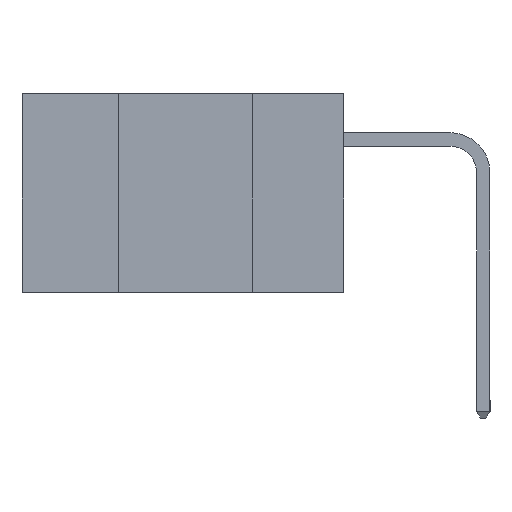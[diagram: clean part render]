
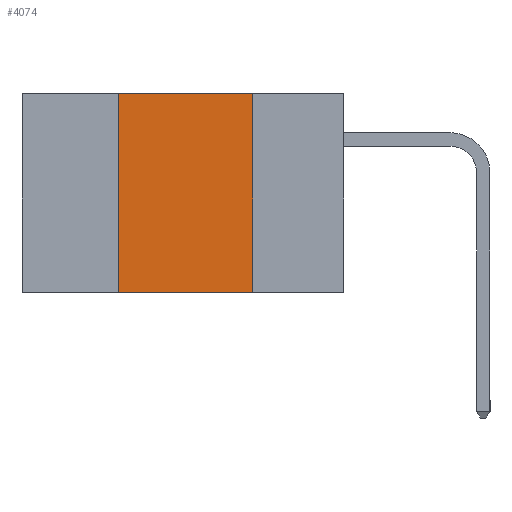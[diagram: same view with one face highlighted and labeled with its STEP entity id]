
A CAD part, left-side view. The second image highlights one B-rep face of the part: STEP entity #4074.
In plain terms, the highlighted planar face has unit normal (-1, 0, 0).
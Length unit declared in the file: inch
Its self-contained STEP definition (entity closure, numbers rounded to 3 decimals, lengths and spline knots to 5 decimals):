
#386 = VECTOR ( 'NONE', #10915, 39.37008 ) ;
#509 = VERTEX_POINT ( 'NONE', #4034 ) ;
#665 = CARTESIAN_POINT ( 'NONE',  ( 0., 0.6, 0. ) ) ;
#705 = ORIENTED_EDGE ( 'NONE', *, *, #10083, .F. ) ;
#811 = VECTOR ( 'NONE', #11705, 39.37008 ) ;
#926 = ORIENTED_EDGE ( 'NONE', *, *, #9241, .F. ) ;
#1350 = LINE ( 'NONE', #15082, #14401 ) ;
#3184 = VERTEX_POINT ( 'NONE', #14435 ) ;
#3360 = EDGE_LOOP ( 'NONE', ( #15332, #705, #926, #4141 ) ) ;
#3818 = LINE ( 'NONE', #4060, #811 ) ;
#4034 = CARTESIAN_POINT ( 'NONE',  ( 0., 0.42, 0. ) ) ;
#4060 = CARTESIAN_POINT ( 'NONE',  ( 0., 0.42, -0.37 ) ) ;
#4074 = ADVANCED_FACE ( 'NONE', ( #5512 ), #8255, .F. ) ;
#4141 = ORIENTED_EDGE ( 'NONE', *, *, #8368, .T. ) ;
#5512 = FACE_OUTER_BOUND ( 'NONE', #3360, .T. ) ;
#5934 = LINE ( 'NONE', #10351, #9000 ) ;
#8171 = DIRECTION ( 'NONE',  ( 0., 0., -1. ) ) ;
#8212 = CARTESIAN_POINT ( 'NONE',  ( 0., 0.17, -0.37 ) ) ;
#8220 = DIRECTION ( 'NONE',  ( 1., 0., 0. ) ) ;
#8255 = PLANE ( 'NONE',  #13648 ) ;
#8330 = CARTESIAN_POINT ( 'NONE',  ( 0., 0.6, 0. ) ) ;
#8368 = EDGE_CURVE ( 'NONE', #15716, #10609, #1350, .T. ) ;
#9000 = VECTOR ( 'NONE', #14012, 39.37008 ) ;
#9241 = EDGE_CURVE ( 'NONE', #15716, #509, #3818, .T. ) ;
#10083 = EDGE_CURVE ( 'NONE', #509, #3184, #16271, .T. ) ;
#10351 = CARTESIAN_POINT ( 'NONE',  ( 0., 0.17, -0.37 ) ) ;
#10609 = VERTEX_POINT ( 'NONE', #8212 ) ;
#10915 = DIRECTION ( 'NONE',  ( 0., -1., 0. ) ) ;
#11705 = DIRECTION ( 'NONE',  ( 0., 0., 1. ) ) ;
#11728 = EDGE_CURVE ( 'NONE', #3184, #10609, #5934, .T. ) ;
#12817 = CARTESIAN_POINT ( 'NONE',  ( 0., 0.42, -0.37 ) ) ;
#13648 = AXIS2_PLACEMENT_3D ( 'NONE', #8330, #8220, #8171 ) ;
#13872 = DIRECTION ( 'NONE',  ( 0., -1., 0. ) ) ;
#14012 = DIRECTION ( 'NONE',  ( 0., 0., -1. ) ) ;
#14401 = VECTOR ( 'NONE', #13872, 39.37008 ) ;
#14435 = CARTESIAN_POINT ( 'NONE',  ( 0., 0.17, 0. ) ) ;
#15082 = CARTESIAN_POINT ( 'NONE',  ( 0., 0.6, -0.37 ) ) ;
#15332 = ORIENTED_EDGE ( 'NONE', *, *, #11728, .F. ) ;
#15716 = VERTEX_POINT ( 'NONE', #12817 ) ;
#16271 = LINE ( 'NONE', #665, #386 ) ;
